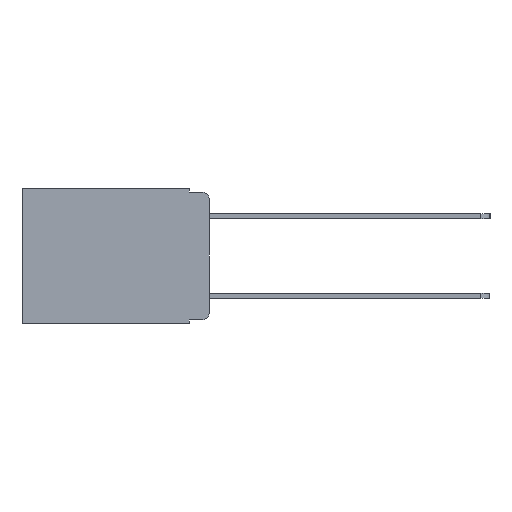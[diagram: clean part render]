
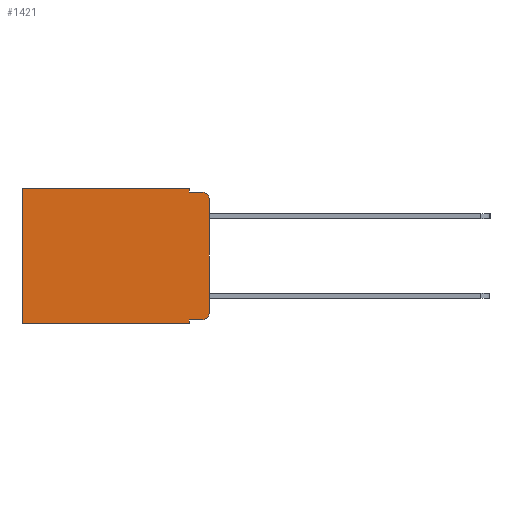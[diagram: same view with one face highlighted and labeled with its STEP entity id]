
A CAD part, left-side view. The second image highlights one B-rep face of the part: STEP entity #1421.
In plain terms, the highlighted planar face has unit normal (-1, 0, 0).
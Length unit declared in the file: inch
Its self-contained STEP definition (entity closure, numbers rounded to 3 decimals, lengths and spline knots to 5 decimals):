
#213 = LINE ( 'NONE', #4769, #7784 ) ;
#1066 = AXIS2_PLACEMENT_3D ( 'NONE', #6474, #16588, #7941 ) ;
#1356 = CARTESIAN_POINT ( 'NONE',  ( 0.298, 0.473, -0.343 ) ) ;
#1421 = ADVANCED_FACE ( 'NONE', ( #12822 ), #4798, .F. ) ;
#1443 = VERTEX_POINT ( 'NONE', #17896 ) ;
#1459 = ORIENTED_EDGE ( 'NONE', *, *, #14738, .F. ) ;
#1540 = EDGE_CURVE ( 'NONE', #16374, #5934, #14418, .T. ) ;
#2090 = VERTEX_POINT ( 'NONE', #13721 ) ;
#2613 = VECTOR ( 'NONE', #18033, 39.37008 ) ;
#2674 = VECTOR ( 'NONE', #16687, 39.37008 ) ;
#2761 = LINE ( 'NONE', #14389, #17364 ) ;
#2969 = EDGE_CURVE ( 'NONE', #14346, #6105, #10504, .T. ) ;
#4038 = ORIENTED_EDGE ( 'NONE', *, *, #17606, .F. ) ;
#4188 = DIRECTION ( 'NONE',  ( 0., 0., -1. ) ) ;
#4369 = ORIENTED_EDGE ( 'NONE', *, *, #14221, .T. ) ;
#4769 = CARTESIAN_POINT ( 'NONE',  ( 0.298, 0.051, 0. ) ) ;
#4798 = PLANE ( 'NONE',  #17133 ) ;
#4952 = CARTESIAN_POINT ( 'NONE',  ( 0.298, 0.051, -0.01 ) ) ;
#5769 = LINE ( 'NONE', #7489, #16865 ) ;
#5934 = VERTEX_POINT ( 'NONE', #15482 ) ;
#5984 = CARTESIAN_POINT ( 'NONE',  ( 0.298, 0.02, -0.313 ) ) ;
#6067 = VERTEX_POINT ( 'NONE', #15661 ) ;
#6105 = VERTEX_POINT ( 'NONE', #10020 ) ;
#6111 = VECTOR ( 'NONE', #10470, 39.37008 ) ;
#6236 = ORIENTED_EDGE ( 'NONE', *, *, #6965, .T. ) ;
#6261 = DIRECTION ( 'NONE',  ( 0., 0., -1. ) ) ;
#6474 = CARTESIAN_POINT ( 'NONE',  ( 0.298, 0.02, -0.03 ) ) ;
#6702 = ORIENTED_EDGE ( 'NONE', *, *, #13741, .F. ) ;
#6877 = ORIENTED_EDGE ( 'NONE', *, *, #1540, .T. ) ;
#6965 = EDGE_CURVE ( 'NONE', #6067, #6105, #13776, .T. ) ;
#7215 = CIRCLE ( 'NONE', #13748, 0.02 ) ;
#7458 = DIRECTION ( 'NONE',  ( 0., 0., -1. ) ) ;
#7489 = CARTESIAN_POINT ( 'NONE',  ( 0.298, 0.473, 0. ) ) ;
#7491 = ORIENTED_EDGE ( 'NONE', *, *, #12758, .T. ) ;
#7784 = VECTOR ( 'NONE', #6261, 39.37008 ) ;
#7886 = CARTESIAN_POINT ( 'NONE',  ( 0.298, 0., 0. ) ) ;
#7941 = DIRECTION ( 'NONE',  ( 0., 0., -1. ) ) ;
#8963 = DIRECTION ( 'NONE',  ( 0., 0., -1. ) ) ;
#9635 = LINE ( 'NONE', #7886, #13880 ) ;
#9981 = LINE ( 'NONE', #14792, #6111 ) ;
#10020 = CARTESIAN_POINT ( 'NONE',  ( 0.298, 0.02, -0.01 ) ) ;
#10402 = CARTESIAN_POINT ( 'NONE',  ( 0.298, 0.051, -0.333 ) ) ;
#10470 = DIRECTION ( 'NONE',  ( 0., 1., 0. ) ) ;
#10504 = LINE ( 'NONE', #4952, #2674 ) ;
#10656 = CARTESIAN_POINT ( 'NONE',  ( 0.298, 0., 0. ) ) ;
#10718 = DIRECTION ( 'NONE',  ( 0., 0., -1. ) ) ;
#11672 = EDGE_CURVE ( 'NONE', #2090, #15317, #9981, .T. ) ;
#12758 = EDGE_CURVE ( 'NONE', #15738, #15317, #5769, .T. ) ;
#12822 = FACE_OUTER_BOUND ( 'NONE', #12871, .T. ) ;
#12871 = EDGE_LOOP ( 'NONE', ( #4038, #6236, #17304, #6702, #18633, #7491, #13706, #1459, #6877, #4369 ) ) ;
#13706 = ORIENTED_EDGE ( 'NONE', *, *, #11672, .F. ) ;
#13721 = CARTESIAN_POINT ( 'NONE',  ( 0.298, 0.051, -0.343 ) ) ;
#13741 = EDGE_CURVE ( 'NONE', #1443, #14346, #213, .T. ) ;
#13748 = AXIS2_PLACEMENT_3D ( 'NONE', #5984, #16126, #7458 ) ;
#13776 = CIRCLE ( 'NONE', #1066, 0.02 ) ;
#13880 = VECTOR ( 'NONE', #17958, 39.37008 ) ;
#13945 = VECTOR ( 'NONE', #16797, 39.37008 ) ;
#14030 = CARTESIAN_POINT ( 'NONE',  ( 0.298, 0.473, 0. ) ) ;
#14221 = EDGE_CURVE ( 'NONE', #5934, #18772, #7215, .T. ) ;
#14346 = VERTEX_POINT ( 'NONE', #16302 ) ;
#14389 = CARTESIAN_POINT ( 'NONE',  ( 0.298, 0.051, 0. ) ) ;
#14418 = LINE ( 'NONE', #18202, #13945 ) ;
#14738 = EDGE_CURVE ( 'NONE', #16374, #2090, #2761, .T. ) ;
#14764 = LINE ( 'NONE', #16626, #2613 ) ;
#14792 = CARTESIAN_POINT ( 'NONE',  ( 0.298, 0., -0.343 ) ) ;
#15317 = VERTEX_POINT ( 'NONE', #1356 ) ;
#15482 = CARTESIAN_POINT ( 'NONE',  ( 0.298, 0.02, -0.333 ) ) ;
#15661 = CARTESIAN_POINT ( 'NONE',  ( 0.298, 0., -0.03 ) ) ;
#15738 = VERTEX_POINT ( 'NONE', #14030 ) ;
#16126 = DIRECTION ( 'NONE',  ( -1., 0., 0. ) ) ;
#16302 = CARTESIAN_POINT ( 'NONE',  ( 0.298, 0.051, -0.01 ) ) ;
#16374 = VERTEX_POINT ( 'NONE', #10402 ) ;
#16472 = EDGE_CURVE ( 'NONE', #1443, #15738, #9635, .T. ) ;
#16480 = DIRECTION ( 'NONE',  ( 1., 0., 0. ) ) ;
#16588 = DIRECTION ( 'NONE',  ( -1., 0., 0. ) ) ;
#16626 = CARTESIAN_POINT ( 'NONE',  ( 0.298, 0., 0. ) ) ;
#16687 = DIRECTION ( 'NONE',  ( 0., -1., 0. ) ) ;
#16797 = DIRECTION ( 'NONE',  ( 0., -1., 0. ) ) ;
#16865 = VECTOR ( 'NONE', #8963, 39.37008 ) ;
#17133 = AXIS2_PLACEMENT_3D ( 'NONE', #10656, #16480, #10718 ) ;
#17304 = ORIENTED_EDGE ( 'NONE', *, *, #2969, .F. ) ;
#17364 = VECTOR ( 'NONE', #4188, 39.37008 ) ;
#17606 = EDGE_CURVE ( 'NONE', #6067, #18772, #14764, .T. ) ;
#17896 = CARTESIAN_POINT ( 'NONE',  ( 0.298, 0.051, 0. ) ) ;
#17958 = DIRECTION ( 'NONE',  ( 0., 1., 0. ) ) ;
#18033 = DIRECTION ( 'NONE',  ( 0., 0., -1. ) ) ;
#18202 = CARTESIAN_POINT ( 'NONE',  ( 0.298, 0.051, -0.333 ) ) ;
#18403 = CARTESIAN_POINT ( 'NONE',  ( 0.298, 0., -0.313 ) ) ;
#18633 = ORIENTED_EDGE ( 'NONE', *, *, #16472, .T. ) ;
#18772 = VERTEX_POINT ( 'NONE', #18403 ) ;
